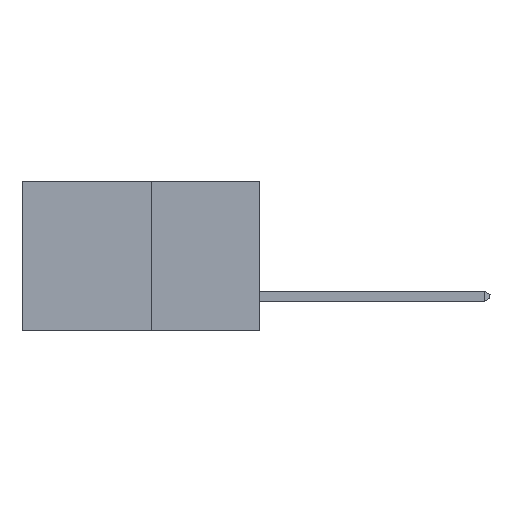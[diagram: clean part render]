
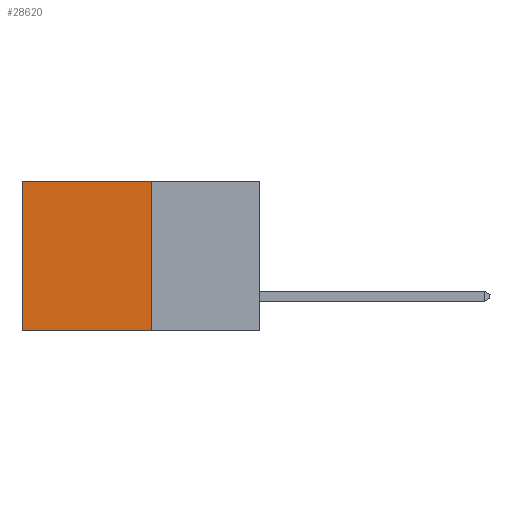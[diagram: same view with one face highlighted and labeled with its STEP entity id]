
A CAD part, left-side view. The second image highlights one B-rep face of the part: STEP entity #28620.
In plain terms, the highlighted planar face has unit normal (-1, 0, 0).
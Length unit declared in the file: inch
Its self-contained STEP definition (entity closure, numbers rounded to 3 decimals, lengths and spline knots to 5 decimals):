
#1524 = ORIENTED_EDGE ( 'NONE', *, *, #3376, .F. ) ;
#1736 = DIRECTION ( 'NONE',  ( 0., 0., -1. ) ) ;
#1749 = AXIS2_PLACEMENT_3D ( 'NONE', #19033, #13936, #32123 ) ;
#1791 = CARTESIAN_POINT ( 'NONE',  ( 0.277, 0.27, -0.37 ) ) ;
#1980 = FACE_OUTER_BOUND ( 'NONE', #26948, .T. ) ;
#3376 = EDGE_CURVE ( 'NONE', #17768, #8554, #31170, .T. ) ;
#5872 = CARTESIAN_POINT ( 'NONE',  ( 0.277, 0.27, 0. ) ) ;
#7027 = CARTESIAN_POINT ( 'NONE',  ( 0.277, 0.27, -0.37 ) ) ;
#8554 = VERTEX_POINT ( 'NONE', #1791 ) ;
#10387 = VERTEX_POINT ( 'NONE', #19504 ) ;
#13325 = CARTESIAN_POINT ( 'NONE',  ( 0.277, 0.59, 0. ) ) ;
#13853 = ORIENTED_EDGE ( 'NONE', *, *, #31600, .T. ) ;
#13936 = DIRECTION ( 'NONE',  ( 1., 0., 0. ) ) ;
#14031 = ORIENTED_EDGE ( 'NONE', *, *, #30572, .T. ) ;
#15716 = CARTESIAN_POINT ( 'NONE',  ( 0.277, 0.27, 0. ) ) ;
#17768 = VERTEX_POINT ( 'NONE', #15716 ) ;
#18449 = VECTOR ( 'NONE', #20060, 39.37008 ) ;
#19033 = CARTESIAN_POINT ( 'NONE',  ( 0.277, 0.27, -0.37 ) ) ;
#19504 = CARTESIAN_POINT ( 'NONE',  ( 0.277, 0.59, -0.37 ) ) ;
#19607 = LINE ( 'NONE', #5872, #33426 ) ;
#20060 = DIRECTION ( 'NONE',  ( 0., 1., 0. ) ) ;
#20647 = EDGE_CURVE ( 'NONE', #8554, #10387, #27039, .T. ) ;
#22911 = DIRECTION ( 'NONE',  ( 0., 0., -1. ) ) ;
#23108 = CARTESIAN_POINT ( 'NONE',  ( 0.277, 0.27, -0.37 ) ) ;
#24177 = DIRECTION ( 'NONE',  ( 0., 1., 0. ) ) ;
#24263 = VECTOR ( 'NONE', #22911, 39.37008 ) ;
#26616 = VECTOR ( 'NONE', #1736, 39.37008 ) ;
#26948 = EDGE_LOOP ( 'NONE', ( #13853, #32729, #1524, #14031 ) ) ;
#27039 = LINE ( 'NONE', #7027, #18449 ) ;
#28620 = ADVANCED_FACE ( 'NONE', ( #1980 ), #29551, .F. ) ;
#29551 = PLANE ( 'NONE',  #1749 ) ;
#30572 = EDGE_CURVE ( 'NONE', #17768, #33745, #19607, .T. ) ;
#31170 = LINE ( 'NONE', #23108, #24263 ) ;
#31600 = EDGE_CURVE ( 'NONE', #33745, #10387, #33492, .T. ) ;
#32123 = DIRECTION ( 'NONE',  ( 0., 0., -1. ) ) ;
#32729 = ORIENTED_EDGE ( 'NONE', *, *, #20647, .F. ) ;
#33127 = CARTESIAN_POINT ( 'NONE',  ( 0.277, 0.59, -0.37 ) ) ;
#33426 = VECTOR ( 'NONE', #24177, 39.37008 ) ;
#33492 = LINE ( 'NONE', #33127, #26616 ) ;
#33745 = VERTEX_POINT ( 'NONE', #13325 ) ;
